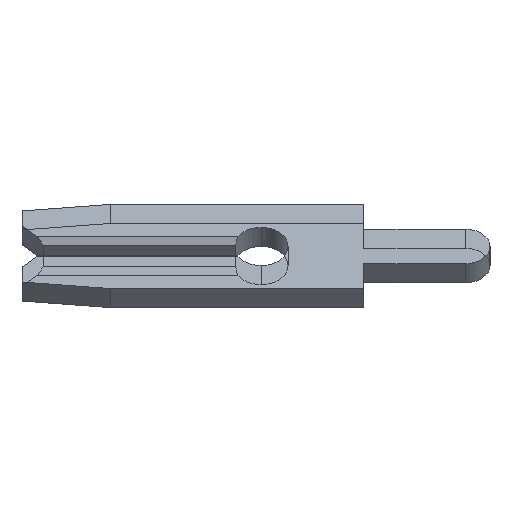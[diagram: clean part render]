
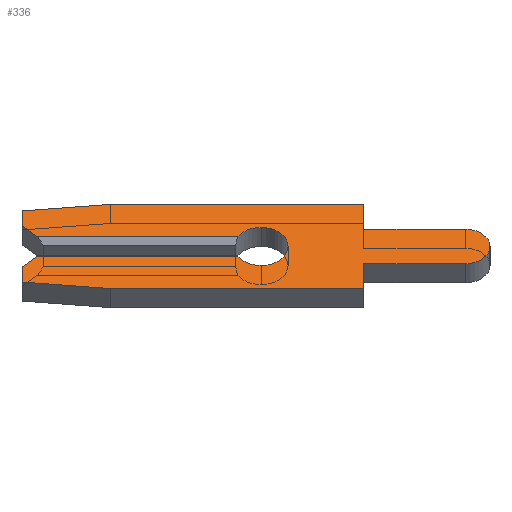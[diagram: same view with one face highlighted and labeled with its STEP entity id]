
A CAD part, left-side view. The second image highlights one B-rep face of the part: STEP entity #336.
In plain terms, the highlighted face is planar.
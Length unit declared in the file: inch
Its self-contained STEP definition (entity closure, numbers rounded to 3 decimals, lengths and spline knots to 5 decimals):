
#6 = VERTEX_POINT ( 'NONE', #2523 ) ;
#35 = VECTOR ( 'NONE', #600, 39.37008 ) ;
#51 = ORIENTED_EDGE ( 'NONE', *, *, #895, .F. ) ;
#143 = LINE ( 'NONE', #1888, #1914 ) ;
#158 = EDGE_CURVE ( 'NONE', #1177, #2045, #185, .T. ) ;
#182 = LINE ( 'NONE', #559, #1475 ) ;
#185 = LINE ( 'NONE', #1034, #2011 ) ;
#207 = CARTESIAN_POINT ( 'NONE',  ( -0.013, 0.146, -0.0575 ) ) ;
#215 = EDGE_CURVE ( 'NONE', #2553, #2469, #1750, .T. ) ;
#216 = VECTOR ( 'NONE', #1195, 39.37008 ) ;
#219 = ORIENTED_EDGE ( 'NONE', *, *, #1051, .F. ) ;
#220 = VERTEX_POINT ( 'NONE', #1261 ) ;
#228 = CARTESIAN_POINT ( 'NONE',  ( -0.013, 0.02252, -0.013 ) ) ;
#239 = CARTESIAN_POINT ( 'NONE',  ( -0.013, -0.1975, 0. ) ) ;
#265 = DIRECTION ( 'NONE',  ( 0., 0., -1. ) ) ;
#273 = DIRECTION ( 'NONE',  ( -1., 0., 0. ) ) ;
#297 = AXIS2_PLACEMENT_3D ( 'NONE', #318, #352, #1891 ) ;
#318 = CARTESIAN_POINT ( 'NONE',  ( -0.013, 0., 0. ) ) ;
#336 = ADVANCED_FACE ( 'NONE', ( #1206 ), #646, .F. ) ;
#352 = DIRECTION ( 'NONE',  ( -1., 0., 0. ) ) ;
#361 = VERTEX_POINT ( 'NONE', #1551 ) ;
#396 = DIRECTION ( 'NONE',  ( 1., 0., 0. ) ) ;
#406 = VERTEX_POINT ( 'NONE', #654 ) ;
#413 = CARTESIAN_POINT ( 'NONE',  ( -0.013, 0., -0.013 ) ) ;
#447 = DIRECTION ( 'NONE',  ( -1., 0., 0. ) ) ;
#452 = ORIENTED_EDGE ( 'NONE', *, *, #2371, .F. ) ;
#460 = EDGE_LOOP ( 'NONE', ( #715, #1009, #51, #1552, #1367, #2022, #219, #898, #2153, #1229, #1122, #1480, #1484, #1883, #750, #1381, #452, #2048 ) ) ;
#500 = VERTEX_POINT ( 'NONE', #1385 ) ;
#526 = CARTESIAN_POINT ( 'NONE',  ( -0.013, -0.099, 0.0235 ) ) ;
#529 = EDGE_CURVE ( 'NONE', #406, #6, #2009, .T. ) ;
#559 = CARTESIAN_POINT ( 'NONE',  ( -0.013, 0.2105, 0.0075 ) ) ;
#587 = AXIS2_PLACEMENT_3D ( 'NONE', #2193, #396, #1578 ) ;
#597 = CARTESIAN_POINT ( 'NONE',  ( -0.013, -0.099, -0.0235 ) ) ;
#600 = DIRECTION ( 'NONE',  ( 0., 0.995, 0.105 ) ) ;
#615 = LINE ( 'NONE', #1075, #1779 ) ;
#625 = EDGE_CURVE ( 'NONE', #500, #1087, #650, .T. ) ;
#646 = PLANE ( 'NONE',  #587 ) ;
#650 = LINE ( 'NONE', #1145, #1226 ) ;
#654 = CARTESIAN_POINT ( 'NONE',  ( -0.013, -0.1975, 0.0235 ) ) ;
#686 = VECTOR ( 'NONE', #1443, 39.37008 ) ;
#693 = CARTESIAN_POINT ( 'NONE',  ( -0.013, -0.099, -0.0575 ) ) ;
#715 = ORIENTED_EDGE ( 'NONE', *, *, #2120, .T. ) ;
#718 = CARTESIAN_POINT ( 'NONE',  ( -0.013, -0.099, -0.0235 ) ) ;
#724 = LINE ( 'NONE', #1017, #942 ) ;
#750 = ORIENTED_EDGE ( 'NONE', *, *, #2692, .F. ) ;
#813 = DIRECTION ( 'NONE',  ( 0., -1., 0. ) ) ;
#871 = CARTESIAN_POINT ( 'NONE',  ( -0.013, -0.099, -0.0575 ) ) ;
#895 = EDGE_CURVE ( 'NONE', #361, #220, #2436, .T. ) ;
#898 = ORIENTED_EDGE ( 'NONE', *, *, #215, .F. ) ;
#906 = VECTOR ( 'NONE', #2410, 39.37008 ) ;
#937 = EDGE_CURVE ( 'NONE', #1114, #1604, #1944, .T. ) ;
#942 = VECTOR ( 'NONE', #1460, 39.37008 ) ;
#1009 = ORIENTED_EDGE ( 'NONE', *, *, #1734, .F. ) ;
#1013 = LINE ( 'NONE', #2483, #216 ) ;
#1017 = CARTESIAN_POINT ( 'NONE',  ( -0.013, -0.099, 0.0575 ) ) ;
#1028 = CARTESIAN_POINT ( 'NONE',  ( -0.013, 0.231, -0.04857 ) ) ;
#1034 = CARTESIAN_POINT ( 'NONE',  ( -0.013, 0.2105, -0.0075 ) ) ;
#1050 = VECTOR ( 'NONE', #1408, 39.37008 ) ;
#1051 = EDGE_CURVE ( 'NONE', #2469, #1177, #1013, .T. ) ;
#1052 = VECTOR ( 'NONE', #1720, 39.37008 ) ;
#1075 = CARTESIAN_POINT ( 'NONE',  ( -0.013, 0.146, 0.0575 ) ) ;
#1087 = VERTEX_POINT ( 'NONE', #1643 ) ;
#1114 = VERTEX_POINT ( 'NONE', #718 ) ;
#1121 = LINE ( 'NONE', #413, #2467 ) ;
#1122 = ORIENTED_EDGE ( 'NONE', *, *, #1547, .F. ) ;
#1130 = AXIS2_PLACEMENT_3D ( 'NONE', #1403, #273, #265 ) ;
#1145 = CARTESIAN_POINT ( 'NONE',  ( -0.013, 0.231, 0.04857 ) ) ;
#1177 = VERTEX_POINT ( 'NONE', #1671 ) ;
#1195 = DIRECTION ( 'NONE',  ( 0., 0., 1. ) ) ;
#1196 = EDGE_CURVE ( 'NONE', #1916, #361, #1882, .T. ) ;
#1206 = FACE_OUTER_BOUND ( 'NONE', #460, .T. ) ;
#1225 = CARTESIAN_POINT ( 'NONE',  ( -0.013, -0.099, 0.0235 ) ) ;
#1226 = VECTOR ( 'NONE', #2232, 39.37008 ) ;
#1229 = ORIENTED_EDGE ( 'NONE', *, *, #937, .F. ) ;
#1237 = CARTESIAN_POINT ( 'NONE',  ( -0.013, 0.216, 0.013 ) ) ;
#1261 = CARTESIAN_POINT ( 'NONE',  ( -0.013, 0., 0.026 ) ) ;
#1277 = DIRECTION ( 'NONE',  ( 0., -0.707, 0.707 ) ) ;
#1296 = EDGE_CURVE ( 'NONE', #1604, #2553, #1652, .T. ) ;
#1344 = LINE ( 'NONE', #526, #1943 ) ;
#1362 = CIRCLE ( 'NONE', #1864, 0.026 ) ;
#1367 = ORIENTED_EDGE ( 'NONE', *, *, #1389, .F. ) ;
#1371 = DIRECTION ( 'NONE',  ( 0., 0., -1. ) ) ;
#1381 = ORIENTED_EDGE ( 'NONE', *, *, #625, .F. ) ;
#1385 = CARTESIAN_POINT ( 'NONE',  ( -0.013, 0.231, 0.04857 ) ) ;
#1389 = EDGE_CURVE ( 'NONE', #2045, #1916, #1121, .T. ) ;
#1401 = CARTESIAN_POINT ( 'NONE',  ( -0.013, 0., 0. ) ) ;
#1402 = VERTEX_POINT ( 'NONE', #1506 ) ;
#1403 = CARTESIAN_POINT ( 'NONE',  ( -0.013, 0., 0. ) ) ;
#1408 = DIRECTION ( 'NONE',  ( 0., -1., 0. ) ) ;
#1443 = DIRECTION ( 'NONE',  ( 0., 0., -1. ) ) ;
#1449 = CARTESIAN_POINT ( 'NONE',  ( -0.013, 0.216, -0.013 ) ) ;
#1460 = DIRECTION ( 'NONE',  ( 0., 0., -1. ) ) ;
#1474 = DIRECTION ( 'NONE',  ( 0., 0.707, 0.707 ) ) ;
#1475 = VECTOR ( 'NONE', #1474, 39.37008 ) ;
#1480 = ORIENTED_EDGE ( 'NONE', *, *, #529, .F. ) ;
#1484 = ORIENTED_EDGE ( 'NONE', *, *, #2273, .F. ) ;
#1485 = CARTESIAN_POINT ( 'NONE',  ( -0.013, 0.146, -0.0575 ) ) ;
#1506 = CARTESIAN_POINT ( 'NONE',  ( -0.013, 0.231, 0.028 ) ) ;
#1547 = EDGE_CURVE ( 'NONE', #6, #1114, #1583, .T. ) ;
#1551 = CARTESIAN_POINT ( 'NONE',  ( -0.013, 0., -0.026 ) ) ;
#1552 = ORIENTED_EDGE ( 'NONE', *, *, #1196, .F. ) ;
#1578 = DIRECTION ( 'NONE',  ( 0., 0., -1. ) ) ;
#1583 = LINE ( 'NONE', #597, #906 ) ;
#1604 = VERTEX_POINT ( 'NONE', #871 ) ;
#1605 = AXIS2_PLACEMENT_3D ( 'NONE', #239, #2429, #2673 ) ;
#1643 = CARTESIAN_POINT ( 'NONE',  ( -0.013, 0.146, 0.0575 ) ) ;
#1652 = LINE ( 'NONE', #207, #1052 ) ;
#1671 = CARTESIAN_POINT ( 'NONE',  ( -0.013, 0.231, -0.028 ) ) ;
#1679 = CARTESIAN_POINT ( 'NONE',  ( -0.013, 0.231, 0.013 ) ) ;
#1720 = DIRECTION ( 'NONE',  ( 0., 1., 0. ) ) ;
#1734 = EDGE_CURVE ( 'NONE', #220, #2761, #1362, .T. ) ;
#1750 = LINE ( 'NONE', #1937, #35 ) ;
#1779 = VECTOR ( 'NONE', #2162, 39.37008 ) ;
#1864 = AXIS2_PLACEMENT_3D ( 'NONE', #1401, #447, #1371 ) ;
#1882 = CIRCLE ( 'NONE', #297, 0.026 ) ;
#1883 = ORIENTED_EDGE ( 'NONE', *, *, #2585, .F. ) ;
#1888 = CARTESIAN_POINT ( 'NONE',  ( -0.013, 0.231, 0.028 ) ) ;
#1891 = DIRECTION ( 'NONE',  ( 0., 0., -1. ) ) ;
#1914 = VECTOR ( 'NONE', #2545, 39.37008 ) ;
#1916 = VERTEX_POINT ( 'NONE', #228 ) ;
#1937 = CARTESIAN_POINT ( 'NONE',  ( -0.013, 0.231, -0.04857 ) ) ;
#1943 = VECTOR ( 'NONE', #2708, 39.37008 ) ;
#1944 = LINE ( 'NONE', #693, #686 ) ;
#1951 = CARTESIAN_POINT ( 'NONE',  ( -0.013, 0.02252, 0.013 ) ) ;
#2009 = CIRCLE ( 'NONE', #1605, 0.0235 ) ;
#2011 = VECTOR ( 'NONE', #1277, 39.37008 ) ;
#2022 = ORIENTED_EDGE ( 'NONE', *, *, #158, .F. ) ;
#2045 = VERTEX_POINT ( 'NONE', #1449 ) ;
#2048 = ORIENTED_EDGE ( 'NONE', *, *, #2589, .F. ) ;
#2120 = EDGE_CURVE ( 'NONE', #2575, #2761, #2408, .T. ) ;
#2153 = ORIENTED_EDGE ( 'NONE', *, *, #1296, .F. ) ;
#2162 = DIRECTION ( 'NONE',  ( 0., -1., 0. ) ) ;
#2193 = CARTESIAN_POINT ( 'NONE',  ( -0.013, 0., 0. ) ) ;
#2232 = DIRECTION ( 'NONE',  ( 0., -0.995, 0.105 ) ) ;
#2244 = VERTEX_POINT ( 'NONE', #2827 ) ;
#2251 = VERTEX_POINT ( 'NONE', #1225 ) ;
#2273 = EDGE_CURVE ( 'NONE', #2251, #406, #1344, .T. ) ;
#2371 = EDGE_CURVE ( 'NONE', #1402, #500, #143, .T. ) ;
#2408 = LINE ( 'NONE', #1679, #1050 ) ;
#2410 = DIRECTION ( 'NONE',  ( 0., 1., 0. ) ) ;
#2429 = DIRECTION ( 'NONE',  ( 1., 0., 0. ) ) ;
#2436 = CIRCLE ( 'NONE', #1130, 0.026 ) ;
#2467 = VECTOR ( 'NONE', #813, 39.37008 ) ;
#2469 = VERTEX_POINT ( 'NONE', #1028 ) ;
#2483 = CARTESIAN_POINT ( 'NONE',  ( -0.013, 0.231, -0.028 ) ) ;
#2523 = CARTESIAN_POINT ( 'NONE',  ( -0.013, -0.1975, -0.0235 ) ) ;
#2545 = DIRECTION ( 'NONE',  ( 0., 0., 1. ) ) ;
#2553 = VERTEX_POINT ( 'NONE', #1485 ) ;
#2575 = VERTEX_POINT ( 'NONE', #1237 ) ;
#2585 = EDGE_CURVE ( 'NONE', #2244, #2251, #724, .T. ) ;
#2589 = EDGE_CURVE ( 'NONE', #2575, #1402, #182, .T. ) ;
#2673 = DIRECTION ( 'NONE',  ( 0., 0., 1. ) ) ;
#2692 = EDGE_CURVE ( 'NONE', #1087, #2244, #615, .T. ) ;
#2708 = DIRECTION ( 'NONE',  ( 0., -1., 0. ) ) ;
#2761 = VERTEX_POINT ( 'NONE', #1951 ) ;
#2827 = CARTESIAN_POINT ( 'NONE',  ( -0.013, -0.099, 0.0575 ) ) ;
